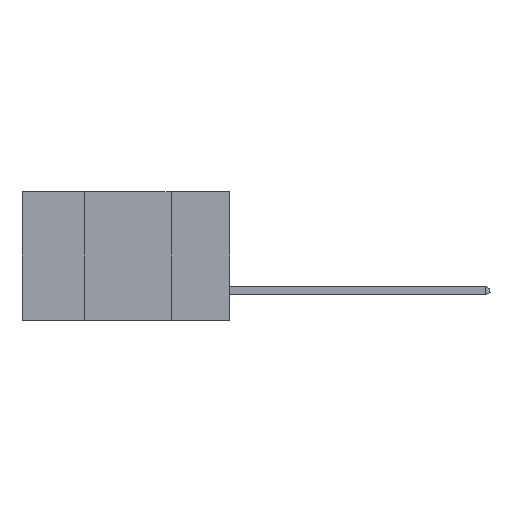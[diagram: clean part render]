
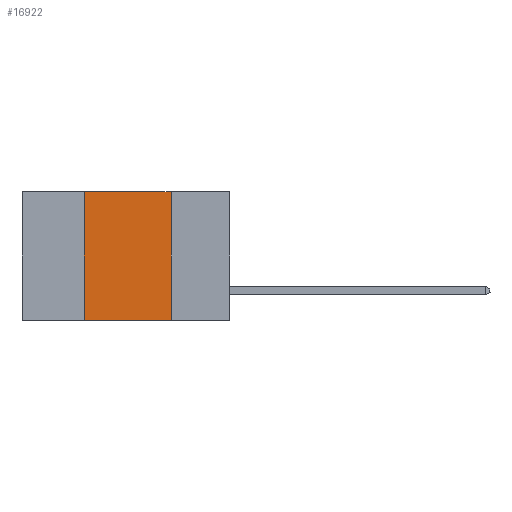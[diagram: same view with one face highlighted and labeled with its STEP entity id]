
A CAD part, left-side view. The second image highlights one B-rep face of the part: STEP entity #16922.
In plain terms, the highlighted planar face has unit normal (-1, 0, 0).
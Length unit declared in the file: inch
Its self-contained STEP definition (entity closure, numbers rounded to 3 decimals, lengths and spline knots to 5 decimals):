
#274 = LINE ( 'NONE', #10082, #8361 ) ;
#1050 = LINE ( 'NONE', #3973, #7198 ) ;
#1362 = DIRECTION ( 'NONE',  ( 1., 0., 0. ) ) ;
#2878 = DIRECTION ( 'NONE',  ( 0., -1., 0. ) ) ;
#3223 = EDGE_CURVE ( 'NONE', #4029, #7600, #11020, .T. ) ;
#3973 = CARTESIAN_POINT ( 'NONE',  ( 0., 0.17, 0. ) ) ;
#4029 = VERTEX_POINT ( 'NONE', #14438 ) ;
#5038 = CARTESIAN_POINT ( 'NONE',  ( 0., 0.6, -0.37 ) ) ;
#5613 = PLANE ( 'NONE',  #19739 ) ;
#6289 = ORIENTED_EDGE ( 'NONE', *, *, #23276, .T. ) ;
#7198 = VECTOR ( 'NONE', #22755, 39.37008 ) ;
#7265 = CARTESIAN_POINT ( 'NONE',  ( 0., 0.42, -0.37 ) ) ;
#7600 = VERTEX_POINT ( 'NONE', #19440 ) ;
#8133 = DIRECTION ( 'NONE',  ( 0., 0., 1. ) ) ;
#8361 = VECTOR ( 'NONE', #8133, 39.37008 ) ;
#8642 = VERTEX_POINT ( 'NONE', #7265 ) ;
#8701 = EDGE_CURVE ( 'NONE', #7600, #26296, #1050, .T. ) ;
#8879 = EDGE_LOOP ( 'NONE', ( #26043, #25003, #18882, #6289 ) ) ;
#9667 = DIRECTION ( 'NONE',  ( 0., -1., 0. ) ) ;
#9809 = DIRECTION ( 'NONE',  ( 0., 0., -1. ) ) ;
#10082 = CARTESIAN_POINT ( 'NONE',  ( 0., 0.42, 0. ) ) ;
#10912 = EDGE_CURVE ( 'NONE', #8642, #4029, #274, .T. ) ;
#11020 = LINE ( 'NONE', #17948, #25412 ) ;
#14438 = CARTESIAN_POINT ( 'NONE',  ( 0., 0.42, 0. ) ) ;
#16342 = VECTOR ( 'NONE', #2878, 39.37008 ) ;
#16922 = ADVANCED_FACE ( 'NONE', ( #20681 ), #5613, .F. ) ;
#17948 = CARTESIAN_POINT ( 'NONE',  ( 0., 0.6, 0. ) ) ;
#18882 = ORIENTED_EDGE ( 'NONE', *, *, #10912, .F. ) ;
#19440 = CARTESIAN_POINT ( 'NONE',  ( 0., 0.17, 0. ) ) ;
#19739 = AXIS2_PLACEMENT_3D ( 'NONE', #20380, #1362, #9809 ) ;
#20380 = CARTESIAN_POINT ( 'NONE',  ( 0., 0.6, 0. ) ) ;
#20520 = CARTESIAN_POINT ( 'NONE',  ( 0., 0.17, -0.37 ) ) ;
#20590 = LINE ( 'NONE', #5038, #16342 ) ;
#20681 = FACE_OUTER_BOUND ( 'NONE', #8879, .T. ) ;
#22755 = DIRECTION ( 'NONE',  ( 0., 0., -1. ) ) ;
#23276 = EDGE_CURVE ( 'NONE', #8642, #26296, #20590, .T. ) ;
#25003 = ORIENTED_EDGE ( 'NONE', *, *, #3223, .F. ) ;
#25412 = VECTOR ( 'NONE', #9667, 39.37008 ) ;
#26043 = ORIENTED_EDGE ( 'NONE', *, *, #8701, .F. ) ;
#26296 = VERTEX_POINT ( 'NONE', #20520 ) ;
